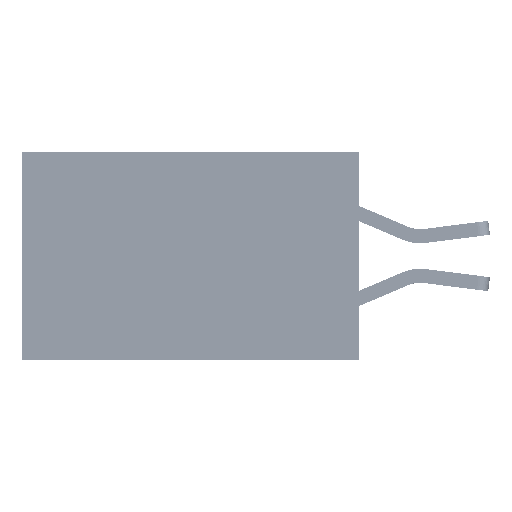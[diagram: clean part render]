
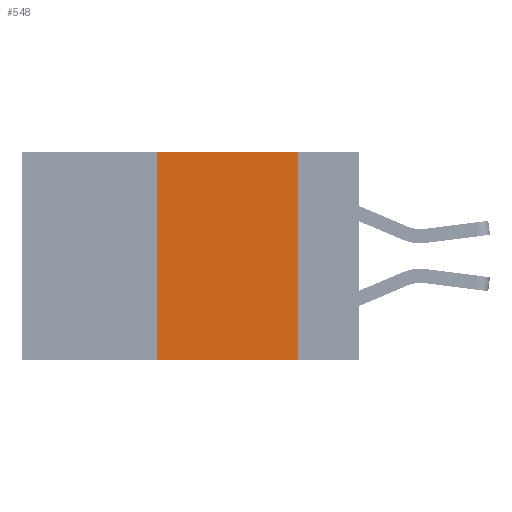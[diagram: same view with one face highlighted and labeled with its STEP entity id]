
A CAD part, left-side view. The second image highlights one B-rep face of the part: STEP entity #548.
In plain terms, the highlighted planar face has unit normal (-1, 0, 0).
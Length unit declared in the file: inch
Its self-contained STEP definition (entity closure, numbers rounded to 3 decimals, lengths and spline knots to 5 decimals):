
#418 = ORIENTED_EDGE ( 'NONE', *, *, #10018, .F. ) ;
#548 = ADVANCED_FACE ( 'NONE', ( #47406 ), #31402, .F. ) ;
#1016 = ORIENTED_EDGE ( 'NONE', *, *, #24367, .T. ) ;
#1146 = CARTESIAN_POINT ( 'NONE',  ( 0., 0.36, -0.37 ) ) ;
#1572 = CARTESIAN_POINT ( 'NONE',  ( 0., 0.36, 0. ) ) ;
#3496 = CARTESIAN_POINT ( 'NONE',  ( 0., 0.6, 0. ) ) ;
#3683 = DIRECTION ( 'NONE',  ( 0., 0., -1. ) ) ;
#3753 = EDGE_CURVE ( 'NONE', #6056, #42840, #48321, .T. ) ;
#6056 = VERTEX_POINT ( 'NONE', #10847 ) ;
#6092 = VECTOR ( 'NONE', #28046, 39.37008 ) ;
#9002 = LINE ( 'NONE', #9229, #19644 ) ;
#9229 = CARTESIAN_POINT ( 'NONE',  ( 0., 0.11, 0. ) ) ;
#10018 = EDGE_CURVE ( 'NONE', #42840, #36209, #9002, .T. ) ;
#10847 = CARTESIAN_POINT ( 'NONE',  ( 0., 0.36, 0. ) ) ;
#11808 = ORIENTED_EDGE ( 'NONE', *, *, #3753, .F. ) ;
#13405 = AXIS2_PLACEMENT_3D ( 'NONE', #3496, #27598, #3683 ) ;
#13734 = DIRECTION ( 'NONE',  ( 0., 0., 1. ) ) ;
#15155 = VERTEX_POINT ( 'NONE', #1146 ) ;
#17585 = VECTOR ( 'NONE', #13734, 39.37008 ) ;
#18530 = CARTESIAN_POINT ( 'NONE',  ( 0., 0.6, -0.37 ) ) ;
#18814 = CARTESIAN_POINT ( 'NONE',  ( 0., 0.11, -0.37 ) ) ;
#19644 = VECTOR ( 'NONE', #48892, 39.37008 ) ;
#24055 = VECTOR ( 'NONE', #50129, 39.37008 ) ;
#24367 = EDGE_CURVE ( 'NONE', #15155, #36209, #34555, .T. ) ;
#24883 = CARTESIAN_POINT ( 'NONE',  ( 0., 0.11, 0. ) ) ;
#27598 = DIRECTION ( 'NONE',  ( 1., 0., 0. ) ) ;
#28046 = DIRECTION ( 'NONE',  ( 0., -1., 0. ) ) ;
#31402 = PLANE ( 'NONE',  #13405 ) ;
#34555 = LINE ( 'NONE', #18530, #24055 ) ;
#36209 = VERTEX_POINT ( 'NONE', #18814 ) ;
#42840 = VERTEX_POINT ( 'NONE', #24883 ) ;
#45532 = EDGE_CURVE ( 'NONE', #15155, #6056, #47853, .T. ) ;
#47406 = FACE_OUTER_BOUND ( 'NONE', #48037, .T. ) ;
#47724 = CARTESIAN_POINT ( 'NONE',  ( 0., 0.6, 0. ) ) ;
#47853 = LINE ( 'NONE', #1572, #17585 ) ;
#48037 = EDGE_LOOP ( 'NONE', ( #418, #11808, #50865, #1016 ) ) ;
#48321 = LINE ( 'NONE', #47724, #6092 ) ;
#48892 = DIRECTION ( 'NONE',  ( 0., 0., -1. ) ) ;
#50129 = DIRECTION ( 'NONE',  ( 0., -1., 0. ) ) ;
#50865 = ORIENTED_EDGE ( 'NONE', *, *, #45532, .F. ) ;
